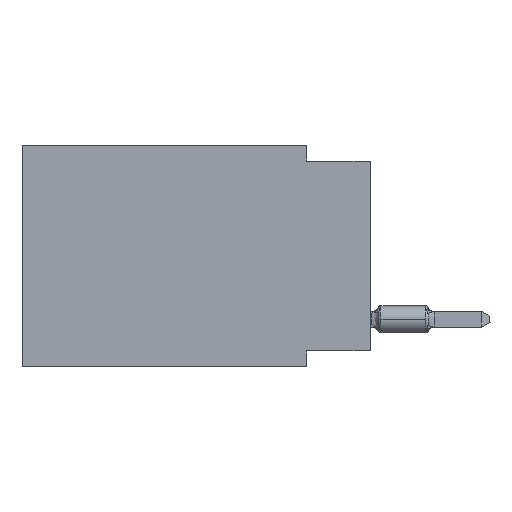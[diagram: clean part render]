
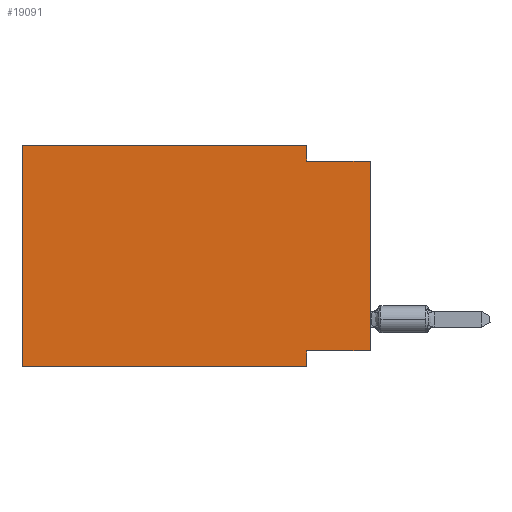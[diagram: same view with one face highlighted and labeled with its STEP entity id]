
A CAD part, left-side view. The second image highlights one B-rep face of the part: STEP entity #19091.
In plain terms, the highlighted planar face has unit normal (-1, 0, 0).
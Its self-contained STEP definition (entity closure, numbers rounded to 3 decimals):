
#830 = DIRECTION ( 'NONE',  ( 0., 0., 1. ) ) ;
#1104 = CARTESIAN_POINT ( 'NONE',  ( 0., 13.97, 0. ) ) ;
#1294 = VERTEX_POINT ( 'NONE', #17653 ) ;
#1331 = VECTOR ( 'NONE', #830, 1000. ) ;
#1747 = ORIENTED_EDGE ( 'NONE', *, *, #32049, .F. ) ;
#1779 = VERTEX_POINT ( 'NONE', #8181 ) ;
#2021 = LINE ( 'NONE', #17129, #18259 ) ;
#2900 = ORIENTED_EDGE ( 'NONE', *, *, #25934, .F. ) ;
#5101 = VECTOR ( 'NONE', #33002, 1000. ) ;
#5625 = VECTOR ( 'NONE', #11026, 1000. ) ;
#5937 = CARTESIAN_POINT ( 'NONE',  ( 0., 13.97, -8.89 ) ) ;
#6155 = CARTESIAN_POINT ( 'NONE',  ( 0., 13.97, -8.89 ) ) ;
#6465 = LINE ( 'NONE', #6629, #19956 ) ;
#6629 = CARTESIAN_POINT ( 'NONE',  ( 0., 2.54, 0. ) ) ;
#6836 = VECTOR ( 'NONE', #10878, 1000. ) ;
#7066 = VECTOR ( 'NONE', #7957, 1000. ) ;
#7388 = VECTOR ( 'NONE', #28140, 1000. ) ;
#7957 = DIRECTION ( 'NONE',  ( 0., 0., -1. ) ) ;
#8181 = CARTESIAN_POINT ( 'NONE',  ( 0., 2.54, -0.635 ) ) ;
#8477 = CARTESIAN_POINT ( 'NONE',  ( 0., 13.97, 0. ) ) ;
#8643 = LINE ( 'NONE', #8477, #1331 ) ;
#8801 = LINE ( 'NONE', #5937, #5625 ) ;
#8901 = EDGE_LOOP ( 'NONE', ( #11731, #13476, #28158, #2900, #15168, #22670, #22858, #1747 ) ) ;
#9633 = VERTEX_POINT ( 'NONE', #24382 ) ;
#10188 = CARTESIAN_POINT ( 'NONE',  ( 0., 0., -8.255 ) ) ;
#10878 = DIRECTION ( 'NONE',  ( 0., -1., 0. ) ) ;
#11026 = DIRECTION ( 'NONE',  ( 0., -1., 0. ) ) ;
#11731 = ORIENTED_EDGE ( 'NONE', *, *, #19405, .T. ) ;
#12269 = EDGE_CURVE ( 'NONE', #16499, #1779, #6465, .T. ) ;
#12506 = CARTESIAN_POINT ( 'NONE',  ( 0., 0., 0. ) ) ;
#13313 = CARTESIAN_POINT ( 'NONE',  ( 0., 2.54, -8.89 ) ) ;
#13475 = EDGE_CURVE ( 'NONE', #9633, #19966, #20665, .T. ) ;
#13476 = ORIENTED_EDGE ( 'NONE', *, *, #32147, .F. ) ;
#13742 = DIRECTION ( 'NONE',  ( 0., 0., -1. ) ) ;
#13769 = CARTESIAN_POINT ( 'NONE',  ( 0., 0., -0.635 ) ) ;
#14115 = DIRECTION ( 'NONE',  ( 0., 0., -1. ) ) ;
#15168 = ORIENTED_EDGE ( 'NONE', *, *, #21028, .F. ) ;
#16499 = VERTEX_POINT ( 'NONE', #20760 ) ;
#17089 = VERTEX_POINT ( 'NONE', #1104 ) ;
#17129 = CARTESIAN_POINT ( 'NONE',  ( 0., 13.97, 0. ) ) ;
#17653 = CARTESIAN_POINT ( 'NONE',  ( 0., 0., -0.635 ) ) ;
#17927 = VERTEX_POINT ( 'NONE', #6155 ) ;
#18159 = LINE ( 'NONE', #10188, #7388 ) ;
#18259 = VECTOR ( 'NONE', #30169, 1000. ) ;
#18272 = EDGE_CURVE ( 'NONE', #17927, #19966, #8801, .T. ) ;
#19091 = ADVANCED_FACE ( 'NONE', ( #31178 ), #20982, .F. ) ;
#19405 = EDGE_CURVE ( 'NONE', #23274, #1294, #30972, .T. ) ;
#19956 = VECTOR ( 'NONE', #14115, 1000. ) ;
#19966 = VERTEX_POINT ( 'NONE', #13313 ) ;
#20665 = LINE ( 'NONE', #33230, #7066 ) ;
#20760 = CARTESIAN_POINT ( 'NONE',  ( 0., 2.54, 0. ) ) ;
#20982 = PLANE ( 'NONE',  #25618 ) ;
#21028 = EDGE_CURVE ( 'NONE', #17927, #17089, #8643, .T. ) ;
#21317 = CARTESIAN_POINT ( 'NONE',  ( 0., 13.97, 0. ) ) ;
#22670 = ORIENTED_EDGE ( 'NONE', *, *, #18272, .T. ) ;
#22858 = ORIENTED_EDGE ( 'NONE', *, *, #13475, .F. ) ;
#23274 = VERTEX_POINT ( 'NONE', #31479 ) ;
#23903 = LINE ( 'NONE', #13769, #6836 ) ;
#24382 = CARTESIAN_POINT ( 'NONE',  ( 0., 2.54, -8.255 ) ) ;
#25618 = AXIS2_PLACEMENT_3D ( 'NONE', #21317, #29310, #13742 ) ;
#25934 = EDGE_CURVE ( 'NONE', #17089, #16499, #2021, .T. ) ;
#28140 = DIRECTION ( 'NONE',  ( 0., 1., 0. ) ) ;
#28158 = ORIENTED_EDGE ( 'NONE', *, *, #12269, .F. ) ;
#29310 = DIRECTION ( 'NONE',  ( 1., 0., 0. ) ) ;
#30169 = DIRECTION ( 'NONE',  ( 0., -1., 0. ) ) ;
#30972 = LINE ( 'NONE', #12506, #5101 ) ;
#31178 = FACE_OUTER_BOUND ( 'NONE', #8901, .T. ) ;
#31479 = CARTESIAN_POINT ( 'NONE',  ( 0., 0., -8.255 ) ) ;
#32049 = EDGE_CURVE ( 'NONE', #23274, #9633, #18159, .T. ) ;
#32147 = EDGE_CURVE ( 'NONE', #1779, #1294, #23903, .T. ) ;
#33002 = DIRECTION ( 'NONE',  ( 0., 0., 1. ) ) ;
#33230 = CARTESIAN_POINT ( 'NONE',  ( 0., 2.54, -8.89 ) ) ;
